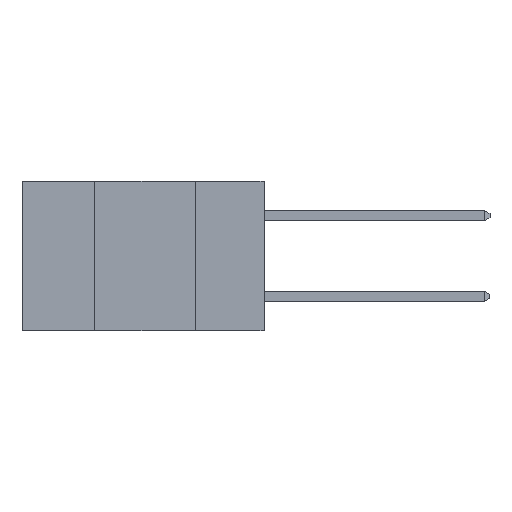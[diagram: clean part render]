
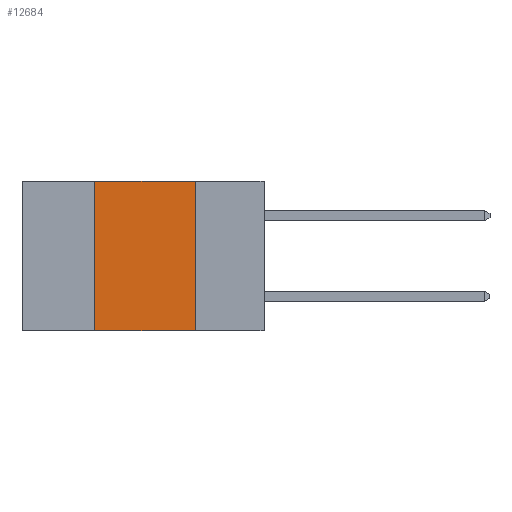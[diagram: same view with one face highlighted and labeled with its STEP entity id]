
A CAD part, left-side view. The second image highlights one B-rep face of the part: STEP entity #12684.
In plain terms, the highlighted planar face has unit normal (-1, 0, 0).
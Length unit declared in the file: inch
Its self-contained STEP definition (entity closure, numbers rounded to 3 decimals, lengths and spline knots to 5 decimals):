
#472 = DIRECTION ( 'NONE',  ( 0., 0., 1. ) ) ;
#666 = ORIENTED_EDGE ( 'NONE', *, *, #11364, .F. ) ;
#3317 = CARTESIAN_POINT ( 'NONE',  ( 0., 0.42, -0.37 ) ) ;
#3423 = ORIENTED_EDGE ( 'NONE', *, *, #9228, .F. ) ;
#4313 = DIRECTION ( 'NONE',  ( 0., -1., 0. ) ) ;
#4410 = VECTOR ( 'NONE', #472, 39.37008 ) ;
#7107 = CARTESIAN_POINT ( 'NONE',  ( 0., 0.42, 0. ) ) ;
#7134 = DIRECTION ( 'NONE',  ( 0., 0., -1. ) ) ;
#7787 = DIRECTION ( 'NONE',  ( 1., 0., 0. ) ) ;
#8100 = VECTOR ( 'NONE', #7134, 39.37008 ) ;
#9228 = EDGE_CURVE ( 'NONE', #12779, #14991, #17646, .T. ) ;
#9488 = DIRECTION ( 'NONE',  ( 0., -1., 0. ) ) ;
#10790 = LINE ( 'NONE', #12705, #14046 ) ;
#11364 = EDGE_CURVE ( 'NONE', #11834, #16102, #13078, .T. ) ;
#11834 = VERTEX_POINT ( 'NONE', #3317 ) ;
#11940 = CARTESIAN_POINT ( 'NONE',  ( 0., 0.17, 0. ) ) ;
#12684 = ADVANCED_FACE ( 'NONE', ( #15488 ), #18928, .F. ) ;
#12705 = CARTESIAN_POINT ( 'NONE',  ( 0., 0.6, 0. ) ) ;
#12779 = VERTEX_POINT ( 'NONE', #12862 ) ;
#12862 = CARTESIAN_POINT ( 'NONE',  ( 0., 0.17, 0. ) ) ;
#13078 = LINE ( 'NONE', #7107, #4410 ) ;
#13991 = CARTESIAN_POINT ( 'NONE',  ( 0., 0.42, 0. ) ) ;
#14038 = CARTESIAN_POINT ( 'NONE',  ( 0., 0.6, -0.37 ) ) ;
#14046 = VECTOR ( 'NONE', #9488, 39.37008 ) ;
#14586 = EDGE_CURVE ( 'NONE', #11834, #14991, #20132, .T. ) ;
#14991 = VERTEX_POINT ( 'NONE', #15218 ) ;
#15218 = CARTESIAN_POINT ( 'NONE',  ( 0., 0.17, -0.37 ) ) ;
#15488 = FACE_OUTER_BOUND ( 'NONE', #20653, .T. ) ;
#15980 = ORIENTED_EDGE ( 'NONE', *, *, #17420, .F. ) ;
#16102 = VERTEX_POINT ( 'NONE', #13991 ) ;
#16464 = VECTOR ( 'NONE', #4313, 39.37008 ) ;
#17420 = EDGE_CURVE ( 'NONE', #16102, #12779, #10790, .T. ) ;
#17428 = CARTESIAN_POINT ( 'NONE',  ( 0., 0.6, 0. ) ) ;
#17646 = LINE ( 'NONE', #11940, #8100 ) ;
#17828 = ORIENTED_EDGE ( 'NONE', *, *, #14586, .T. ) ;
#18928 = PLANE ( 'NONE',  #20005 ) ;
#18988 = DIRECTION ( 'NONE',  ( 0., 0., -1. ) ) ;
#20005 = AXIS2_PLACEMENT_3D ( 'NONE', #17428, #7787, #18988 ) ;
#20132 = LINE ( 'NONE', #14038, #16464 ) ;
#20653 = EDGE_LOOP ( 'NONE', ( #3423, #15980, #666, #17828 ) ) ;
